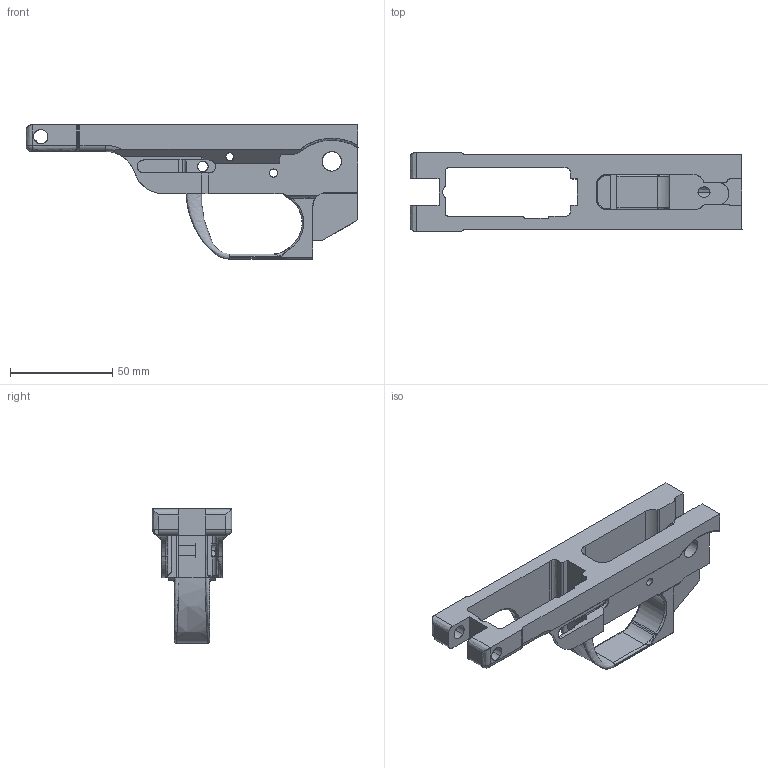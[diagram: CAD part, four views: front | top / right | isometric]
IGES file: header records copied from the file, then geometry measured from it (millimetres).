
Start section: SolidWorks IGES file using analytic representation for surfaces
Global section: file name: Phobos_V1.2_Front.IGS; native system: SolidWorks 2015; preprocessor: SolidWorks 2015; author: WarFairy; date: 150521.091041; units: inch
Bounding box: 162.67 x 39 x 65.79 mm (x, y, z)
Surface area: 33167.5 mm2 (no closed solid volume)
Topology: 0 solids, 0 shells, 282 faces, 3335 edges, 3328 vertices
Faces by surface type: bspline 146, revolution 136
